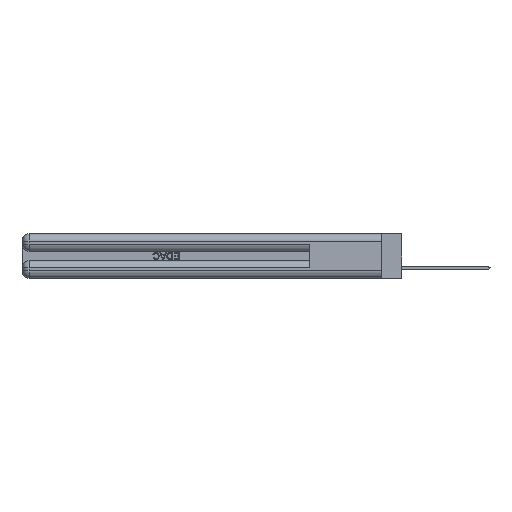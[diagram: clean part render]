
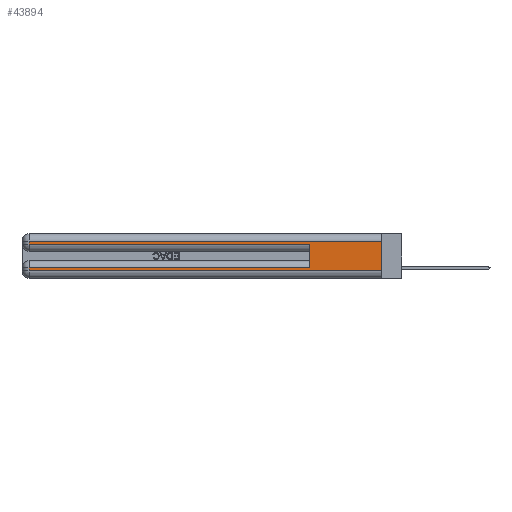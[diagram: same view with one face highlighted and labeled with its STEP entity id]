
A CAD part, left-side view. The second image highlights one B-rep face of the part: STEP entity #43894.
In plain terms, the highlighted planar face has unit normal (-1, 0, 0).
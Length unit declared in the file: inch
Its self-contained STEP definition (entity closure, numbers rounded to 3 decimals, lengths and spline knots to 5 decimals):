
#124 = CARTESIAN_POINT ( 'NONE',  ( 0., 0.6, 0.285 ) ) ;
#1150 = DIRECTION ( 'NONE',  ( 0., -1., 0. ) ) ;
#1260 = EDGE_CURVE ( 'NONE', #28993, #31553, #9819, .T. ) ;
#2151 = EDGE_LOOP ( 'NONE', ( #35921, #36806, #17492, #27700, #19677, #10403, #35026, #36001 ) ) ;
#5124 = EDGE_CURVE ( 'NONE', #47512, #43154, #43184, .T. ) ;
#6222 = LINE ( 'NONE', #47078, #47782 ) ;
#6349 = DIRECTION ( 'NONE',  ( 0., 0., -1. ) ) ;
#6520 = DIRECTION ( 'NONE',  ( 1., 0., 0. ) ) ;
#7106 = LINE ( 'NONE', #32941, #45719 ) ;
#9637 = VECTOR ( 'NONE', #1150, 39.37008 ) ;
#9819 = LINE ( 'NONE', #30574, #31451 ) ;
#10403 = ORIENTED_EDGE ( 'NONE', *, *, #19040, .T. ) ;
#10617 = EDGE_CURVE ( 'NONE', #17621, #25382, #42216, .T. ) ;
#10921 = CARTESIAN_POINT ( 'NONE',  ( 0., 0., 0.37 ) ) ;
#13180 = DIRECTION ( 'NONE',  ( 0., 1., 0. ) ) ;
#13672 = CARTESIAN_POINT ( 'NONE',  ( 0., 0., 0.37 ) ) ;
#13883 = VERTEX_POINT ( 'NONE', #18489 ) ;
#14609 = CARTESIAN_POINT ( 'NONE',  ( 0., 0.6, 0.085 ) ) ;
#16941 = EDGE_CURVE ( 'NONE', #45657, #43154, #29311, .T. ) ;
#17492 = ORIENTED_EDGE ( 'NONE', *, *, #10617, .T. ) ;
#17621 = VERTEX_POINT ( 'NONE', #41721 ) ;
#17809 = CARTESIAN_POINT ( 'NONE',  ( 0., 0., 0.06 ) ) ;
#18149 = VECTOR ( 'NONE', #22480, 39.37008 ) ;
#18489 = CARTESIAN_POINT ( 'NONE',  ( 0., 2.94, 0.085 ) ) ;
#18549 = DIRECTION ( 'NONE',  ( 0., 0., -1. ) ) ;
#19040 = EDGE_CURVE ( 'NONE', #28993, #13883, #6222, .T. ) ;
#19677 = ORIENTED_EDGE ( 'NONE', *, *, #1260, .F. ) ;
#20315 = EDGE_CURVE ( 'NONE', #47512, #17621, #7106, .T. ) ;
#20793 = VECTOR ( 'NONE', #34326, 39.37008 ) ;
#22480 = DIRECTION ( 'NONE',  ( 0., -1., 0. ) ) ;
#23042 = CARTESIAN_POINT ( 'NONE',  ( 0., 0., 0.285 ) ) ;
#23924 = EDGE_CURVE ( 'NONE', #13883, #45657, #36092, .T. ) ;
#24192 = CARTESIAN_POINT ( 'NONE',  ( 0., 0., 0.31 ) ) ;
#25382 = VERTEX_POINT ( 'NONE', #34548 ) ;
#27700 = ORIENTED_EDGE ( 'NONE', *, *, #33425, .T. ) ;
#28993 = VERTEX_POINT ( 'NONE', #14609 ) ;
#29311 = LINE ( 'NONE', #37353, #18149 ) ;
#30139 = DIRECTION ( 'NONE',  ( 0., 0., 1. ) ) ;
#30574 = CARTESIAN_POINT ( 'NONE',  ( 0., 0.6, 0.145 ) ) ;
#31451 = VECTOR ( 'NONE', #30139, 39.37008 ) ;
#31553 = VERTEX_POINT ( 'NONE', #124 ) ;
#32399 = PLANE ( 'NONE',  #33076 ) ;
#32941 = CARTESIAN_POINT ( 'NONE',  ( 0., 0., 0.31 ) ) ;
#33076 = AXIS2_PLACEMENT_3D ( 'NONE', #13672, #6520, #6349 ) ;
#33425 = EDGE_CURVE ( 'NONE', #25382, #31553, #38294, .T. ) ;
#33737 = CARTESIAN_POINT ( 'NONE',  ( 0., 2.94, 0.06 ) ) ;
#34326 = DIRECTION ( 'NONE',  ( 0., 0., -1. ) ) ;
#34389 = CARTESIAN_POINT ( 'NONE',  ( 0., 2.94, 0.37 ) ) ;
#34548 = CARTESIAN_POINT ( 'NONE',  ( 0., 2.94, 0.285 ) ) ;
#35026 = ORIENTED_EDGE ( 'NONE', *, *, #23924, .T. ) ;
#35921 = ORIENTED_EDGE ( 'NONE', *, *, #5124, .F. ) ;
#36001 = ORIENTED_EDGE ( 'NONE', *, *, #16941, .T. ) ;
#36092 = LINE ( 'NONE', #45626, #20793 ) ;
#36806 = ORIENTED_EDGE ( 'NONE', *, *, #20315, .T. ) ;
#37353 = CARTESIAN_POINT ( 'NONE',  ( 0., 0., 0.06 ) ) ;
#38194 = DIRECTION ( 'NONE',  ( 0., 0., -1. ) ) ;
#38294 = LINE ( 'NONE', #23042, #9637 ) ;
#41018 = FACE_OUTER_BOUND ( 'NONE', #2151, .T. ) ;
#41721 = CARTESIAN_POINT ( 'NONE',  ( 0., 2.94, 0.31 ) ) ;
#42216 = LINE ( 'NONE', #34389, #45717 ) ;
#43154 = VERTEX_POINT ( 'NONE', #17809 ) ;
#43184 = LINE ( 'NONE', #10921, #44352 ) ;
#43894 = ADVANCED_FACE ( 'NONE', ( #41018 ), #32399, .F. ) ;
#44218 = DIRECTION ( 'NONE',  ( 0., 1., 0. ) ) ;
#44352 = VECTOR ( 'NONE', #18549, 39.37008 ) ;
#45626 = CARTESIAN_POINT ( 'NONE',  ( 0., 2.94, 0.37 ) ) ;
#45657 = VERTEX_POINT ( 'NONE', #33737 ) ;
#45717 = VECTOR ( 'NONE', #38194, 39.37008 ) ;
#45719 = VECTOR ( 'NONE', #44218, 39.37008 ) ;
#47078 = CARTESIAN_POINT ( 'NONE',  ( 0., 0., 0.085 ) ) ;
#47512 = VERTEX_POINT ( 'NONE', #24192 ) ;
#47782 = VECTOR ( 'NONE', #13180, 39.37008 ) ;
